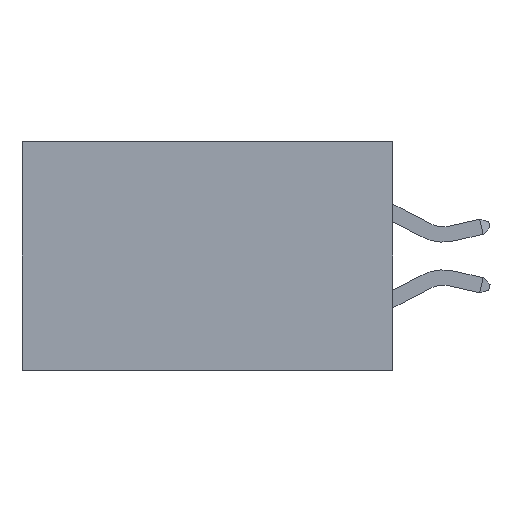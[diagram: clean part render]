
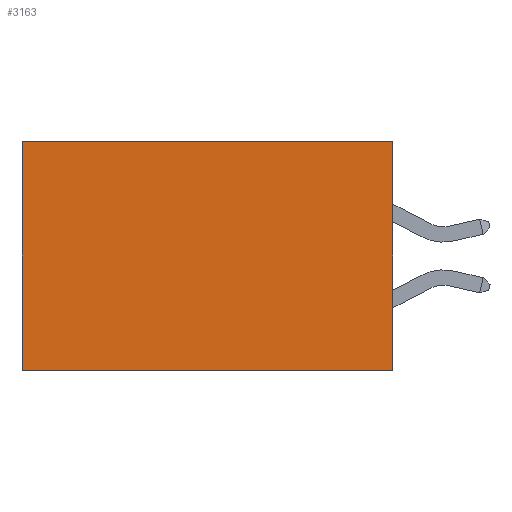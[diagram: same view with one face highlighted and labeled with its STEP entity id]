
A CAD part, left-side view. The second image highlights one B-rep face of the part: STEP entity #3163.
In plain terms, the highlighted planar face has unit normal (-1, 0, 0).
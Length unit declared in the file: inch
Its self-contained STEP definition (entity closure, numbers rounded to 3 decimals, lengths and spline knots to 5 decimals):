
#375 = CARTESIAN_POINT ( 'NONE',  ( 0.2875, 0., 0. ) ) ;
#638 = DIRECTION ( 'NONE',  ( 0., 0., -1. ) ) ;
#1118 = CARTESIAN_POINT ( 'NONE',  ( 0.2875, 0., 0. ) ) ;
#1335 = DIRECTION ( 'NONE',  ( 1., 0., 0. ) ) ;
#1676 = DIRECTION ( 'NONE',  ( 0., 0., -1. ) ) ;
#2147 = CARTESIAN_POINT ( 'NONE',  ( 0.2875, 0.6, 0. ) ) ;
#2162 = CARTESIAN_POINT ( 'NONE',  ( 0.2875, 0., 0. ) ) ;
#2260 = VERTEX_POINT ( 'NONE', #10733 ) ;
#2956 = EDGE_CURVE ( 'NONE', #6585, #8784, #7491, .T. ) ;
#3163 = ADVANCED_FACE ( 'NONE', ( #21404 ), #3474, .F. ) ;
#3351 = DIRECTION ( 'NONE',  ( 0., 1., 0. ) ) ;
#3474 = PLANE ( 'NONE',  #21728 ) ;
#4232 = CARTESIAN_POINT ( 'NONE',  ( 0.2875, 0.6, 0. ) ) ;
#5132 = VECTOR ( 'NONE', #3351, 39.37008 ) ;
#5392 = ORIENTED_EDGE ( 'NONE', *, *, #7365, .T. ) ;
#6585 = VERTEX_POINT ( 'NONE', #4232 ) ;
#7170 = EDGE_CURVE ( 'NONE', #2260, #8784, #17863, .T. ) ;
#7365 = EDGE_CURVE ( 'NONE', #12079, #6585, #18399, .T. ) ;
#7491 = LINE ( 'NONE', #2147, #11392 ) ;
#7950 = ORIENTED_EDGE ( 'NONE', *, *, #2956, .T. ) ;
#8531 = ORIENTED_EDGE ( 'NONE', *, *, #19328, .F. ) ;
#8784 = VERTEX_POINT ( 'NONE', #20232 ) ;
#9074 = DIRECTION ( 'NONE',  ( 0., 0., -1. ) ) ;
#10733 = CARTESIAN_POINT ( 'NONE',  ( 0.2875, 0., -0.37 ) ) ;
#11392 = VECTOR ( 'NONE', #1676, 39.37008 ) ;
#11678 = CARTESIAN_POINT ( 'NONE',  ( 0.2875, 0., 0. ) ) ;
#12079 = VERTEX_POINT ( 'NONE', #1118 ) ;
#12100 = EDGE_LOOP ( 'NONE', ( #7950, #14490, #8531, #5392 ) ) ;
#12986 = CARTESIAN_POINT ( 'NONE',  ( 0.2875, 0., -0.37 ) ) ;
#12997 = VECTOR ( 'NONE', #14641, 39.37008 ) ;
#14490 = ORIENTED_EDGE ( 'NONE', *, *, #7170, .F. ) ;
#14641 = DIRECTION ( 'NONE',  ( 0., 1., 0. ) ) ;
#14709 = VECTOR ( 'NONE', #9074, 39.37008 ) ;
#17863 = LINE ( 'NONE', #12986, #12997 ) ;
#18399 = LINE ( 'NONE', #11678, #5132 ) ;
#19044 = LINE ( 'NONE', #2162, #14709 ) ;
#19328 = EDGE_CURVE ( 'NONE', #12079, #2260, #19044, .T. ) ;
#20232 = CARTESIAN_POINT ( 'NONE',  ( 0.2875, 0.6, -0.37 ) ) ;
#21404 = FACE_OUTER_BOUND ( 'NONE', #12100, .T. ) ;
#21728 = AXIS2_PLACEMENT_3D ( 'NONE', #375, #1335, #638 ) ;
